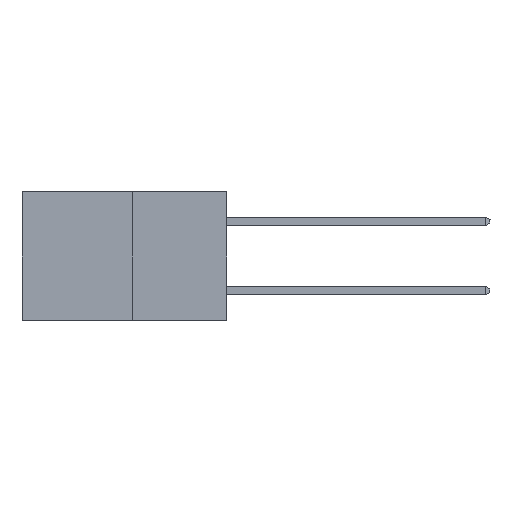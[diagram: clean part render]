
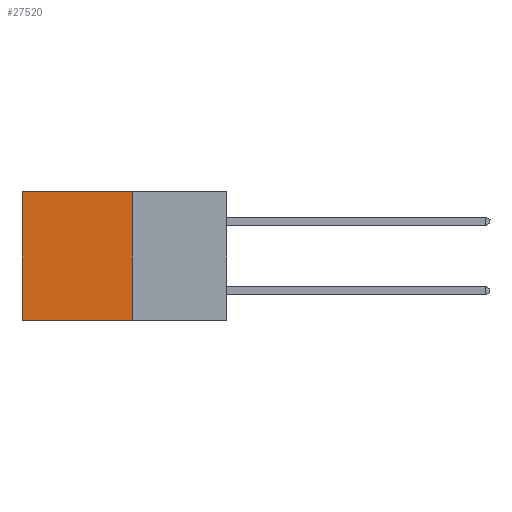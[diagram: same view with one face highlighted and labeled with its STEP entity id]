
A CAD part, left-side view. The second image highlights one B-rep face of the part: STEP entity #27520.
In plain terms, the highlighted planar face has unit normal (-1, 0, 0).
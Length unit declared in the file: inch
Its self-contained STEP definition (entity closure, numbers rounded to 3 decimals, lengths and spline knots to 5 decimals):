
#610 = CARTESIAN_POINT ( 'NONE',  ( 0.277, 0.27, -0.37 ) ) ;
#705 = CARTESIAN_POINT ( 'NONE',  ( 0.277, 0.59, -0.37 ) ) ;
#720 = DIRECTION ( 'NONE',  ( 0., 1., 0. ) ) ;
#1191 = LINE ( 'NONE', #610, #27413 ) ;
#1600 = FACE_OUTER_BOUND ( 'NONE', #4508, .T. ) ;
#2735 = AXIS2_PLACEMENT_3D ( 'NONE', #29592, #13993, #32191 ) ;
#3034 = VERTEX_POINT ( 'NONE', #19531 ) ;
#4508 = EDGE_LOOP ( 'NONE', ( #11985, #30470, #28906, #5425 ) ) ;
#5267 = CARTESIAN_POINT ( 'NONE',  ( 0.277, 0.59, -0.37 ) ) ;
#5425 = ORIENTED_EDGE ( 'NONE', *, *, #33271, .T. ) ;
#6168 = VERTEX_POINT ( 'NONE', #5267 ) ;
#8688 = EDGE_CURVE ( 'NONE', #15659, #26371, #10578, .T. ) ;
#9761 = VECTOR ( 'NONE', #10679, 39.37008 ) ;
#10578 = LINE ( 'NONE', #20992, #9761 ) ;
#10679 = DIRECTION ( 'NONE',  ( 0., 0., -1. ) ) ;
#11360 = PLANE ( 'NONE',  #2735 ) ;
#11929 = VECTOR ( 'NONE', #14747, 39.37008 ) ;
#11985 = ORIENTED_EDGE ( 'NONE', *, *, #30207, .T. ) ;
#13685 = DIRECTION ( 'NONE',  ( 0., 0., -1. ) ) ;
#13993 = DIRECTION ( 'NONE',  ( 1., 0., 0. ) ) ;
#14747 = DIRECTION ( 'NONE',  ( 0., 1., 0. ) ) ;
#15659 = VERTEX_POINT ( 'NONE', #21637 ) ;
#17246 = EDGE_CURVE ( 'NONE', #26371, #6168, #1191, .T. ) ;
#18891 = LINE ( 'NONE', #27729, #11929 ) ;
#19531 = CARTESIAN_POINT ( 'NONE',  ( 0.277, 0.59, 0. ) ) ;
#19651 = CARTESIAN_POINT ( 'NONE',  ( 0.277, 0.27, -0.37 ) ) ;
#20992 = CARTESIAN_POINT ( 'NONE',  ( 0.277, 0.27, -0.37 ) ) ;
#21175 = VECTOR ( 'NONE', #13685, 39.37008 ) ;
#21637 = CARTESIAN_POINT ( 'NONE',  ( 0.277, 0.27, 0. ) ) ;
#22803 = LINE ( 'NONE', #705, #21175 ) ;
#26371 = VERTEX_POINT ( 'NONE', #19651 ) ;
#27413 = VECTOR ( 'NONE', #720, 39.37008 ) ;
#27520 = ADVANCED_FACE ( 'NONE', ( #1600 ), #11360, .F. ) ;
#27729 = CARTESIAN_POINT ( 'NONE',  ( 0.277, 0.27, 0. ) ) ;
#28906 = ORIENTED_EDGE ( 'NONE', *, *, #8688, .F. ) ;
#29592 = CARTESIAN_POINT ( 'NONE',  ( 0.277, 0.27, -0.37 ) ) ;
#30207 = EDGE_CURVE ( 'NONE', #3034, #6168, #22803, .T. ) ;
#30470 = ORIENTED_EDGE ( 'NONE', *, *, #17246, .F. ) ;
#32191 = DIRECTION ( 'NONE',  ( 0., 0., -1. ) ) ;
#33271 = EDGE_CURVE ( 'NONE', #15659, #3034, #18891, .T. ) ;
